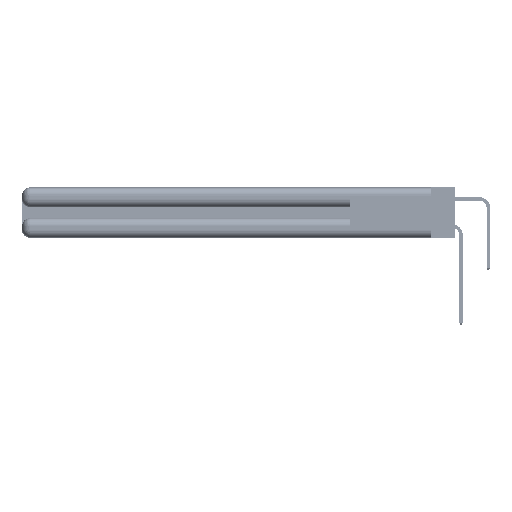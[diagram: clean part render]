
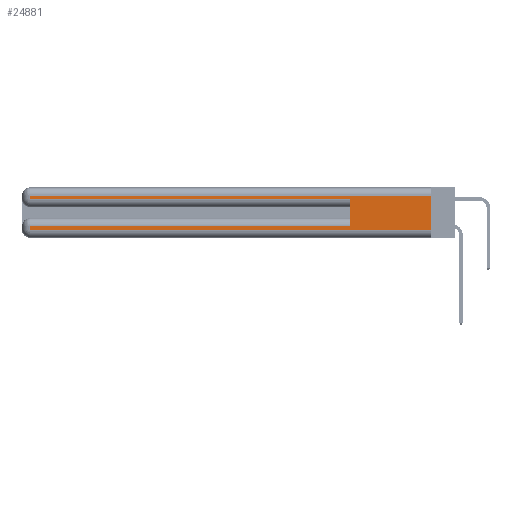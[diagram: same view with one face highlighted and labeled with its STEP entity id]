
A CAD part, left-side view. The second image highlights one B-rep face of the part: STEP entity #24881.
In plain terms, the highlighted planar face has unit normal (-1, 0, 0).
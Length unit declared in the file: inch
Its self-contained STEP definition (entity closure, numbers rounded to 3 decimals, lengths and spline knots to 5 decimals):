
#1857 = EDGE_CURVE ( 'NONE', #43636, #47422, #17128, .T. ) ;
#4388 = CARTESIAN_POINT ( 'NONE',  ( 0., 2.94, 0.31 ) ) ;
#4887 = VERTEX_POINT ( 'NONE', #25187 ) ;
#5048 = DIRECTION ( 'NONE',  ( 0., 0., -1. ) ) ;
#5754 = CARTESIAN_POINT ( 'NONE',  ( 0., 2.94, 0.37 ) ) ;
#6095 = CARTESIAN_POINT ( 'NONE',  ( 0., 0., 0.285 ) ) ;
#6265 = VECTOR ( 'NONE', #35354, 39.37008 ) ;
#7875 = EDGE_CURVE ( 'NONE', #23936, #4887, #46195, .T. ) ;
#8096 = CARTESIAN_POINT ( 'NONE',  ( 0., 0., 0.37 ) ) ;
#8615 = VERTEX_POINT ( 'NONE', #17384 ) ;
#9815 = EDGE_CURVE ( 'NONE', #14608, #32468, #45327, .T. ) ;
#10191 = DIRECTION ( 'NONE',  ( 0., 0., 1. ) ) ;
#10696 = CARTESIAN_POINT ( 'NONE',  ( 0., 2.94, 0.285 ) ) ;
#11586 = ORIENTED_EDGE ( 'NONE', *, *, #28568, .T. ) ;
#14454 = CARTESIAN_POINT ( 'NONE',  ( 0., 0.6, 0.085 ) ) ;
#14608 = VERTEX_POINT ( 'NONE', #4388 ) ;
#14773 = CARTESIAN_POINT ( 'NONE',  ( 0., 2.94, 0.37 ) ) ;
#15401 = ORIENTED_EDGE ( 'NONE', *, *, #16809, .T. ) ;
#16809 = EDGE_CURVE ( 'NONE', #8615, #4887, #41855, .T. ) ;
#17058 = CARTESIAN_POINT ( 'NONE',  ( 0., 0., 0.06 ) ) ;
#17128 = LINE ( 'NONE', #23763, #6265 ) ;
#17384 = CARTESIAN_POINT ( 'NONE',  ( 0., 2.94, 0.06 ) ) ;
#18110 = VECTOR ( 'NONE', #5048, 39.37008 ) ;
#18159 = VECTOR ( 'NONE', #10191, 39.37008 ) ;
#18609 = DIRECTION ( 'NONE',  ( 0., -1., 0. ) ) ;
#19064 = ORIENTED_EDGE ( 'NONE', *, *, #37312, .T. ) ;
#19518 = VECTOR ( 'NONE', #49707, 39.37008 ) ;
#19764 = VECTOR ( 'NONE', #35948, 39.37008 ) ;
#23340 = ORIENTED_EDGE ( 'NONE', *, *, #37287, .T. ) ;
#23763 = CARTESIAN_POINT ( 'NONE',  ( 0., 0., 0.085 ) ) ;
#23884 = LINE ( 'NONE', #42847, #18159 ) ;
#23936 = VERTEX_POINT ( 'NONE', #41243 ) ;
#24575 = DIRECTION ( 'NONE',  ( 0., 0., -1. ) ) ;
#24649 = EDGE_LOOP ( 'NONE', ( #38381, #11586, #36501, #23340, #40194, #32182, #19064, #15401 ) ) ;
#24748 = DIRECTION ( 'NONE',  ( 1., 0., 0. ) ) ;
#24881 = ADVANCED_FACE ( 'NONE', ( #29174 ), #28490, .F. ) ;
#25052 = VECTOR ( 'NONE', #48141, 39.37008 ) ;
#25187 = CARTESIAN_POINT ( 'NONE',  ( 0., 0., 0.06 ) ) ;
#25671 = VECTOR ( 'NONE', #18609, 39.37008 ) ;
#26971 = VECTOR ( 'NONE', #42527, 39.37008 ) ;
#27254 = EDGE_CURVE ( 'NONE', #43636, #41445, #23884, .T. ) ;
#28490 = PLANE ( 'NONE',  #41901 ) ;
#28568 = EDGE_CURVE ( 'NONE', #23936, #14608, #38472, .T. ) ;
#29174 = FACE_OUTER_BOUND ( 'NONE', #24649, .T. ) ;
#29530 = CARTESIAN_POINT ( 'NONE',  ( 0., 0., 0.37 ) ) ;
#32182 = ORIENTED_EDGE ( 'NONE', *, *, #1857, .T. ) ;
#32468 = VERTEX_POINT ( 'NONE', #10696 ) ;
#35354 = DIRECTION ( 'NONE',  ( 0., 1., 0. ) ) ;
#35948 = DIRECTION ( 'NONE',  ( 0., 0., -1. ) ) ;
#36501 = ORIENTED_EDGE ( 'NONE', *, *, #9815, .T. ) ;
#37116 = LINE ( 'NONE', #5754, #26971 ) ;
#37287 = EDGE_CURVE ( 'NONE', #32468, #41445, #42260, .T. ) ;
#37312 = EDGE_CURVE ( 'NONE', #47422, #8615, #37116, .T. ) ;
#38381 = ORIENTED_EDGE ( 'NONE', *, *, #7875, .F. ) ;
#38472 = LINE ( 'NONE', #39569, #25052 ) ;
#39334 = CARTESIAN_POINT ( 'NONE',  ( 0., 2.94, 0.085 ) ) ;
#39569 = CARTESIAN_POINT ( 'NONE',  ( 0., 0., 0.31 ) ) ;
#40194 = ORIENTED_EDGE ( 'NONE', *, *, #27254, .F. ) ;
#41243 = CARTESIAN_POINT ( 'NONE',  ( 0., 0., 0.31 ) ) ;
#41445 = VERTEX_POINT ( 'NONE', #50703 ) ;
#41855 = LINE ( 'NONE', #17058, #19518 ) ;
#41901 = AXIS2_PLACEMENT_3D ( 'NONE', #8096, #24748, #24575 ) ;
#42260 = LINE ( 'NONE', #6095, #25671 ) ;
#42527 = DIRECTION ( 'NONE',  ( 0., 0., -1. ) ) ;
#42847 = CARTESIAN_POINT ( 'NONE',  ( 0., 0.6, 0.145 ) ) ;
#43636 = VERTEX_POINT ( 'NONE', #14454 ) ;
#45327 = LINE ( 'NONE', #14773, #19764 ) ;
#46195 = LINE ( 'NONE', #29530, #18110 ) ;
#47422 = VERTEX_POINT ( 'NONE', #39334 ) ;
#48141 = DIRECTION ( 'NONE',  ( 0., 1., 0. ) ) ;
#49707 = DIRECTION ( 'NONE',  ( 0., -1., 0. ) ) ;
#50703 = CARTESIAN_POINT ( 'NONE',  ( 0., 0.6, 0.285 ) ) ;
